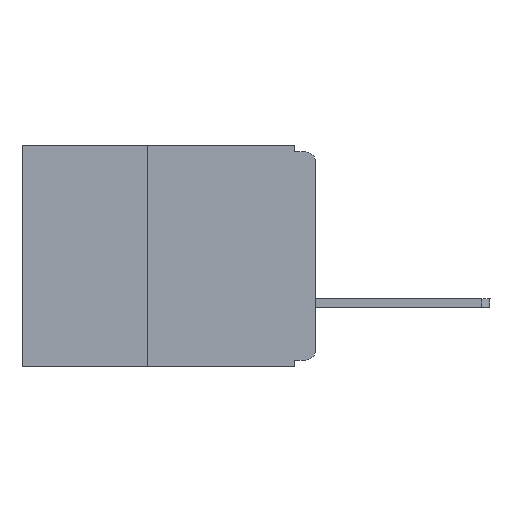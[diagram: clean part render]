
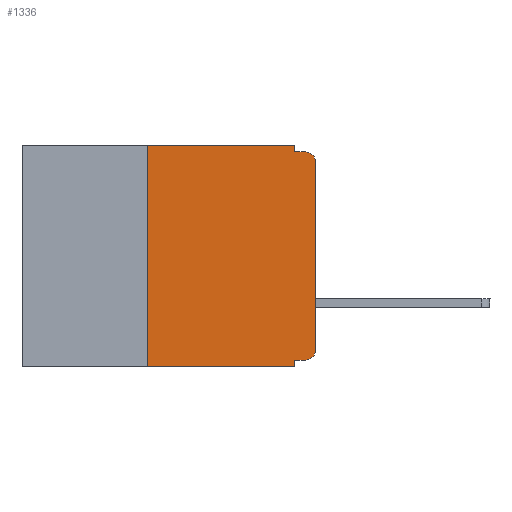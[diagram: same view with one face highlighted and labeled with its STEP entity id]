
A CAD part, left-side view. The second image highlights one B-rep face of the part: STEP entity #1336.
In plain terms, the highlighted planar face has unit normal (-1, 0, 0).
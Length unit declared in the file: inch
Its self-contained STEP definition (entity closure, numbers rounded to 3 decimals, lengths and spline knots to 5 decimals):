
#66 = CARTESIAN_POINT ( 'NONE',  ( 0., 0.031, -0.33 ) ) ;
#120 = DIRECTION ( 'NONE',  ( 0., 0., -1. ) ) ;
#284 = LINE ( 'NONE', #3662, #12015 ) ;
#295 = LINE ( 'NONE', #12002, #298 ) ;
#298 = VECTOR ( 'NONE', #6307, 39.37008 ) ;
#301 = CARTESIAN_POINT ( 'NONE',  ( 0., 0.015, -0.025 ) ) ;
#505 = ORIENTED_EDGE ( 'NONE', *, *, #7018, .F. ) ;
#682 = ORIENTED_EDGE ( 'NONE', *, *, #2097, .T. ) ;
#692 = CARTESIAN_POINT ( 'NONE',  ( 0., 0.031, -0.33 ) ) ;
#956 = ORIENTED_EDGE ( 'NONE', *, *, #7037, .F. ) ;
#1062 = VERTEX_POINT ( 'NONE', #2290 ) ;
#1178 = VECTOR ( 'NONE', #5748, 39.37008 ) ;
#1218 = FACE_OUTER_BOUND ( 'NONE', #4371, .T. ) ;
#1305 = DIRECTION ( 'NONE',  ( 0., 0., -1. ) ) ;
#1310 = ORIENTED_EDGE ( 'NONE', *, *, #2942, .T. ) ;
#1336 = ADVANCED_FACE ( 'NONE', ( #1218 ), #3487, .F. ) ;
#1376 = EDGE_CURVE ( 'NONE', #1062, #5469, #5836, .T. ) ;
#1520 = VERTEX_POINT ( 'NONE', #2522 ) ;
#1632 = AXIS2_PLACEMENT_3D ( 'NONE', #301, #8561, #1305 ) ;
#1828 = ORIENTED_EDGE ( 'NONE', *, *, #7323, .T. ) ;
#1921 = DIRECTION ( 'NONE',  ( 0., 1., 0. ) ) ;
#2097 = EDGE_CURVE ( 'NONE', #5469, #7014, #7841, .T. ) ;
#2154 = ORIENTED_EDGE ( 'NONE', *, *, #6420, .F. ) ;
#2290 = CARTESIAN_POINT ( 'NONE',  ( 0., 0.015, -0.32 ) ) ;
#2338 = EDGE_CURVE ( 'NONE', #2485, #3405, #10020, .T. ) ;
#2415 = DIRECTION ( 'NONE',  ( 0., -1., 0. ) ) ;
#2485 = VERTEX_POINT ( 'NONE', #4161 ) ;
#2522 = CARTESIAN_POINT ( 'NONE',  ( 0., 0.25, -0.33 ) ) ;
#2700 = CARTESIAN_POINT ( 'NONE',  ( 0., 0., -0.025 ) ) ;
#2829 = CARTESIAN_POINT ( 'NONE',  ( 0., 0.015, -0.305 ) ) ;
#2942 = EDGE_CURVE ( 'NONE', #1520, #3074, #8533, .T. ) ;
#3074 = VERTEX_POINT ( 'NONE', #692 ) ;
#3094 = VECTOR ( 'NONE', #4168, 39.37008 ) ;
#3276 = CARTESIAN_POINT ( 'NONE',  ( 0., 0., -0.305 ) ) ;
#3405 = VERTEX_POINT ( 'NONE', #4530 ) ;
#3487 = PLANE ( 'NONE',  #9683 ) ;
#3662 = CARTESIAN_POINT ( 'NONE',  ( 0., 0., -0.32 ) ) ;
#4042 = CARTESIAN_POINT ( 'NONE',  ( 0., 0., 0. ) ) ;
#4090 = EDGE_CURVE ( 'NONE', #1062, #7727, #284, .T. ) ;
#4097 = VECTOR ( 'NONE', #2415, 39.37008 ) ;
#4156 = ORIENTED_EDGE ( 'NONE', *, *, #5352, .F. ) ;
#4161 = CARTESIAN_POINT ( 'NONE',  ( 0., 0.25, 0. ) ) ;
#4168 = DIRECTION ( 'NONE',  ( 0., 0., 1. ) ) ;
#4371 = EDGE_LOOP ( 'NONE', ( #682, #1828, #505, #2154, #11361, #956, #1310, #4156, #8947, #9306 ) ) ;
#4395 = CARTESIAN_POINT ( 'NONE',  ( 0., 0.437, 0. ) ) ;
#4530 = CARTESIAN_POINT ( 'NONE',  ( 0., 0.031, 0. ) ) ;
#4565 = DIRECTION ( 'NONE',  ( 0., 0., -1. ) ) ;
#4628 = DIRECTION ( 'NONE',  ( 0., -1., 0. ) ) ;
#4866 = LINE ( 'NONE', #10099, #9178 ) ;
#5352 = EDGE_CURVE ( 'NONE', #7727, #3074, #5465, .T. ) ;
#5465 = LINE ( 'NONE', #66, #7907 ) ;
#5469 = VERTEX_POINT ( 'NONE', #3276 ) ;
#5748 = DIRECTION ( 'NONE',  ( 0., -1., 0. ) ) ;
#5836 = CIRCLE ( 'NONE', #9276, 0.015 ) ;
#5962 = CARTESIAN_POINT ( 'NONE',  ( 0., 0.031, -0.01 ) ) ;
#6213 = VECTOR ( 'NONE', #4628, 39.37008 ) ;
#6307 = DIRECTION ( 'NONE',  ( 0., 0., 1. ) ) ;
#6420 = EDGE_CURVE ( 'NONE', #3405, #10645, #4866, .T. ) ;
#6504 = DIRECTION ( 'NONE',  ( 0., 0., -1. ) ) ;
#6713 = CIRCLE ( 'NONE', #1632, 0.015 ) ;
#7014 = VERTEX_POINT ( 'NONE', #2700 ) ;
#7018 = EDGE_CURVE ( 'NONE', #10645, #9605, #10192, .T. ) ;
#7037 = EDGE_CURVE ( 'NONE', #1520, #2485, #295, .T. ) ;
#7323 = EDGE_CURVE ( 'NONE', #7014, #9605, #6713, .T. ) ;
#7407 = DIRECTION ( 'NONE',  ( 1., 0., 0. ) ) ;
#7727 = VERTEX_POINT ( 'NONE', #10219 ) ;
#7841 = LINE ( 'NONE', #4042, #3094 ) ;
#7907 = VECTOR ( 'NONE', #6504, 39.37008 ) ;
#8533 = LINE ( 'NONE', #11345, #1178 ) ;
#8561 = DIRECTION ( 'NONE',  ( -1., 0., 0. ) ) ;
#8947 = ORIENTED_EDGE ( 'NONE', *, *, #4090, .F. ) ;
#9178 = VECTOR ( 'NONE', #4565, 39.37008 ) ;
#9184 = CARTESIAN_POINT ( 'NONE',  ( 0., 0.437, 0. ) ) ;
#9276 = AXIS2_PLACEMENT_3D ( 'NONE', #2829, #10173, #120 ) ;
#9302 = DIRECTION ( 'NONE',  ( 0., 0., -1. ) ) ;
#9306 = ORIENTED_EDGE ( 'NONE', *, *, #1376, .T. ) ;
#9605 = VERTEX_POINT ( 'NONE', #11928 ) ;
#9683 = AXIS2_PLACEMENT_3D ( 'NONE', #9184, #7407, #9302 ) ;
#10020 = LINE ( 'NONE', #4395, #4097 ) ;
#10099 = CARTESIAN_POINT ( 'NONE',  ( 0., 0.031, 0. ) ) ;
#10173 = DIRECTION ( 'NONE',  ( -1., 0., 0. ) ) ;
#10192 = LINE ( 'NONE', #11890, #6213 ) ;
#10219 = CARTESIAN_POINT ( 'NONE',  ( 0., 0.031, -0.32 ) ) ;
#10645 = VERTEX_POINT ( 'NONE', #5962 ) ;
#11345 = CARTESIAN_POINT ( 'NONE',  ( 0., 0.437, -0.33 ) ) ;
#11361 = ORIENTED_EDGE ( 'NONE', *, *, #2338, .F. ) ;
#11890 = CARTESIAN_POINT ( 'NONE',  ( 0., 0., -0.01 ) ) ;
#11928 = CARTESIAN_POINT ( 'NONE',  ( 0., 0.015, -0.01 ) ) ;
#12002 = CARTESIAN_POINT ( 'NONE',  ( 0., 0.25, -0.33 ) ) ;
#12015 = VECTOR ( 'NONE', #1921, 39.37008 ) ;
